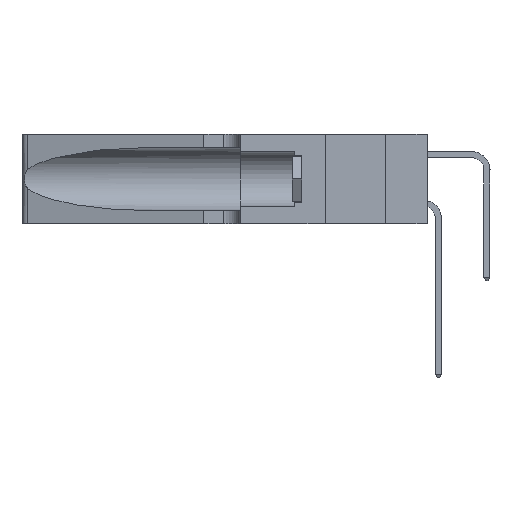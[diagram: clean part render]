
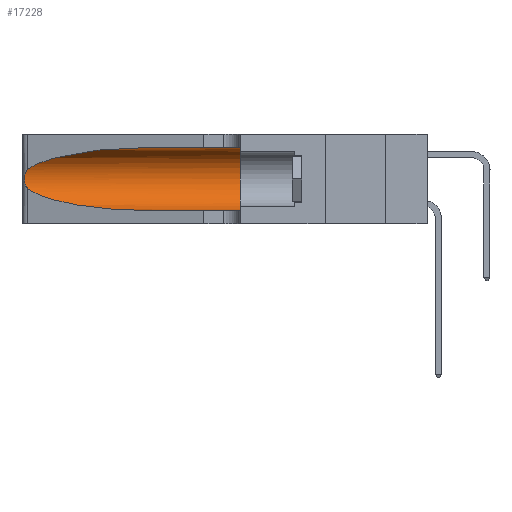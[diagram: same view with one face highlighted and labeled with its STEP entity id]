
A CAD part, left-side view. The second image highlights one B-rep face of the part: STEP entity #17228.
In plain terms, the highlighted cylindrical face has radius 3.308 mm (diameter 6.617 mm), a partial arc.
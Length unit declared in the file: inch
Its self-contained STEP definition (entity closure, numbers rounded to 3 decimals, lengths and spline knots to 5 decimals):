
#45 = CARTESIAN_POINT ( 'NONE',  ( 0.25487, 1.22718, 0.22369 ) ) ;
#126 = EDGE_CURVE ( 'NONE', #3768, #28833, #2221, .T. ) ;
#592 = CARTESIAN_POINT ( 'NONE',  ( 0.1305, 1.61858, 0.31525 ) ) ;
#925 = CARTESIAN_POINT ( 'NONE',  ( 0.2373, 1.15595, 0.28018 ) ) ;
#1068 = CARTESIAN_POINT ( 'NONE',  ( 0.18966, 0.96281, 0.31525 ) ) ;
#1209 = EDGE_CURVE ( 'NONE', #15984, #3768, #41935, .T. ) ;
#2221 = B_SPLINE_CURVE_WITH_KNOTS ( 'NONE', 3,
 ( #45, #33136, #6663, #9543, #36449, #13277, #9952, #32586, #6527, #29259, #29666, #33001, #39461, #31988 ),
 .UNSPECIFIED., .F., .F.,
 ( 4, 2, 2, 2, 2, 2, 4 ),
 ( 0., 0.00027, 0.00053, 0.00107, 0.0016, 0.00187, 0.00214 ),
 .UNSPECIFIED. ) ;
#2738 = CARTESIAN_POINT ( 'NONE',  ( 0.25487, 1.22718, 0.14631 ) ) ;
#3768 = VERTEX_POINT ( 'NONE', #26968 ) ;
#3807 = ORIENTED_EDGE ( 'NONE', *, *, #17010, .F. ) ;
#3946 = CARTESIAN_POINT ( 'NONE',  ( 0.25487, 1.22718, 0.14631 ) ) ;
#4235 = CARTESIAN_POINT ( 'NONE',  ( 0.25487, 1.22718, 0.22369 ) ) ;
#5008 = CARTESIAN_POINT ( 'NONE',  ( 0.1305, 1.61858, 0.05475 ) ) ;
#6527 = CARTESIAN_POINT ( 'NONE',  ( 0.26017, 1.23833, 0.17102 ) ) ;
#6663 = CARTESIAN_POINT ( 'NONE',  ( 0.25639, 1.23184, 0.21858 ) ) ;
#9344 = ORIENTED_EDGE ( 'NONE', *, *, #126, .T. ) ;
#9543 = CARTESIAN_POINT ( 'NONE',  ( 0.25787, 1.23484, 0.2124 ) ) ;
#9952 = CARTESIAN_POINT ( 'NONE',  ( 0.26075, 1.23896, 0.19203 ) ) ;
#11112 = VECTOR ( 'NONE', #29957, 39.37008 ) ;
#12859 = DIRECTION ( 'NONE',  ( 0., 1., 0. ) ) ;
#13161 = VERTEX_POINT ( 'NONE', #32318 ) ;
#13277 = CARTESIAN_POINT ( 'NONE',  ( 0.26018, 1.23835, 0.19895 ) ) ;
#14268 = ORIENTED_EDGE ( 'NONE', *, *, #25090, .T. ) ;
#15464 = DIRECTION ( 'NONE',  ( 0., 0., -1. ) ) ;
#15730 = EDGE_CURVE ( 'NONE', #15984, #13161, #39069, .T. ) ;
#15984 = VERTEX_POINT ( 'NONE', #23885 ) ;
#17010 = EDGE_CURVE ( 'NONE', #13161, #37717, #27564, .T. ) ;
#17221 = AXIS2_PLACEMENT_3D ( 'NONE', #42501, #12859, #29373 ) ;
#17228 = ADVANCED_FACE ( 'NONE', ( #37391 ), #26045, .F. ) ;
#17354 = CARTESIAN_POINT ( 'NONE',  ( 0.1305, 1.61858, 0.185 ) ) ;
#17378 = CARTESIAN_POINT ( 'NONE',  ( 0.1305, 0.72297, 0.31525 ) ) ;
#18664 = AXIS2_PLACEMENT_3D ( 'NONE', #17354, #28667, #15464 ) ;
#20448 = CARTESIAN_POINT ( 'NONE',  ( 0.18966, 0.96281, 0.05475 ) ) ;
#20726 = VERTEX_POINT ( 'NONE', #25210 ) ;
#21146 = ORIENTED_EDGE ( 'NONE', *, *, #1209, .T. ) ;
#23473 = ORIENTED_EDGE ( 'NONE', *, *, #15730, .F. ) ;
#23651 = CARTESIAN_POINT ( 'NONE',  ( 0.2373, 1.15595, 0.08982 ) ) ;
#23885 = CARTESIAN_POINT ( 'NONE',  ( 0.1305, 0.72297, 0.31525 ) ) ;
#23937 = CARTESIAN_POINT ( 'NONE',  ( 0.1305, 0.72297, 0.05475 ) ) ;
#23946 = LINE ( 'NONE', #5008, #29635 ) ;
#25090 = EDGE_CURVE ( 'NONE', #28833, #20726, #31653, .T. ) ;
#25210 = CARTESIAN_POINT ( 'NONE',  ( 0.1305, 0.72297, 0.05475 ) ) ;
#26045 = CYLINDRICAL_SURFACE ( 'NONE', #18664, 0.13025 ) ;
#26672 = EDGE_LOOP ( 'NONE', ( #21146, #9344, #14268, #40085, #3807, #23473 ) ) ;
#26968 = CARTESIAN_POINT ( 'NONE',  ( 0.25487, 1.22718, 0.22369 ) ) ;
#27564 = CIRCLE ( 'NONE', #17221, 0.13025 ) ;
#28159 = DIRECTION ( 'NONE',  ( 0., -1., 0. ) ) ;
#28667 = DIRECTION ( 'NONE',  ( 0., -1., 0. ) ) ;
#28833 = VERTEX_POINT ( 'NONE', #2738 ) ;
#29259 = CARTESIAN_POINT ( 'NONE',  ( 0.25856, 1.23593, 0.16098 ) ) ;
#29373 = DIRECTION ( 'NONE',  ( 0., 0., 1. ) ) ;
#29635 = VECTOR ( 'NONE', #28159, 39.37008 ) ;
#29666 = CARTESIAN_POINT ( 'NONE',  ( 0.25789, 1.23486, 0.15765 ) ) ;
#29957 = DIRECTION ( 'NONE',  ( 0., -1., 0. ) ) ;
#31653 =( BOUNDED_CURVE ( )  B_SPLINE_CURVE ( 3, ( #3946, #23651, #20448, #23937 ),
 .UNSPECIFIED., .F., .T. ) 
 B_SPLINE_CURVE_WITH_KNOTS ( ( 4, 4 ),
 ( 3.44316, 4.71239 ),
 .UNSPECIFIED. ) 
 CURVE ( )  GEOMETRIC_REPRESENTATION_ITEM ( )  RATIONAL_B_SPLINE_CURVE ( ( 1., 0.87, 0.87, 1. ) ) 
 REPRESENTATION_ITEM ( '' )  );
#31988 = CARTESIAN_POINT ( 'NONE',  ( 0.25487, 1.22718, 0.14631 ) ) ;
#32318 = CARTESIAN_POINT ( 'NONE',  ( 0.1305, 0.35, 0.31525 ) ) ;
#32586 = CARTESIAN_POINT ( 'NONE',  ( 0.26075, 1.23896, 0.178 ) ) ;
#32900 = CARTESIAN_POINT ( 'NONE',  ( 0.1305, 0.35, 0.05475 ) ) ;
#33001 = CARTESIAN_POINT ( 'NONE',  ( 0.25639, 1.23186, 0.15144 ) ) ;
#33136 = CARTESIAN_POINT ( 'NONE',  ( 0.25555, 1.22994, 0.2215 ) ) ;
#36449 = CARTESIAN_POINT ( 'NONE',  ( 0.25854, 1.2359, 0.20912 ) ) ;
#37391 = FACE_OUTER_BOUND ( 'NONE', #26672, .T. ) ;
#37717 = VERTEX_POINT ( 'NONE', #32900 ) ;
#39069 = LINE ( 'NONE', #592, #11112 ) ;
#39461 = CARTESIAN_POINT ( 'NONE',  ( 0.25555, 1.22993, 0.14849 ) ) ;
#40085 = ORIENTED_EDGE ( 'NONE', *, *, #41866, .T. ) ;
#41866 = EDGE_CURVE ( 'NONE', #20726, #37717, #23946, .T. ) ;
#41935 =( BOUNDED_CURVE ( )  B_SPLINE_CURVE ( 3, ( #17378, #1068, #925, #4235 ),
 .UNSPECIFIED., .F., .T. ) 
 B_SPLINE_CURVE_WITH_KNOTS ( ( 4, 4 ),
 ( 1.5708, 2.84003 ),
 .UNSPECIFIED. ) 
 CURVE ( )  GEOMETRIC_REPRESENTATION_ITEM ( )  RATIONAL_B_SPLINE_CURVE ( ( 1., 0.87, 0.87, 1. ) ) 
 REPRESENTATION_ITEM ( '' )  );
#42501 = CARTESIAN_POINT ( 'NONE',  ( 0.1305, 0.35, 0.185 ) ) ;
